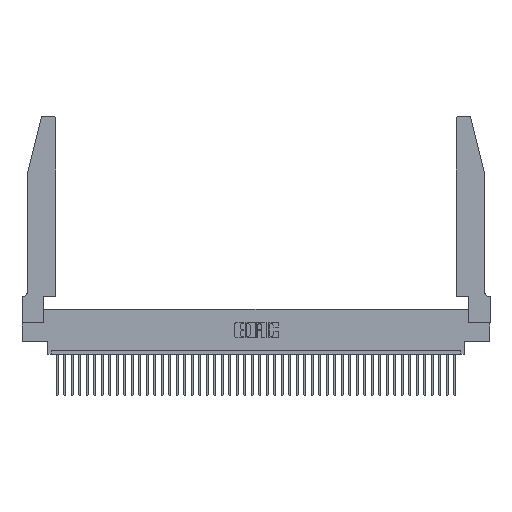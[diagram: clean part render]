
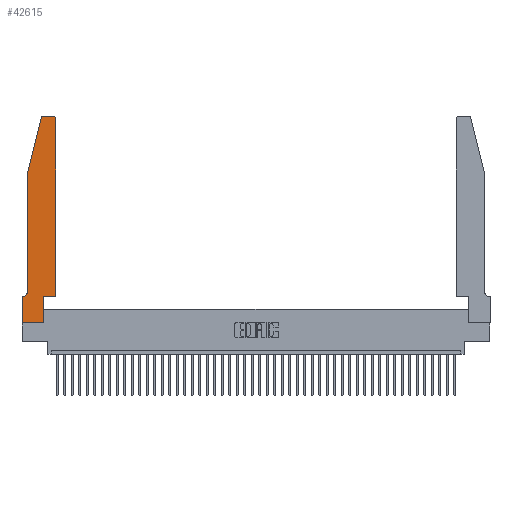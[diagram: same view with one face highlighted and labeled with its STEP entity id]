
A CAD part, top view. The second image highlights one B-rep face of the part: STEP entity #42615.
In plain terms, the highlighted planar face has unit normal (0, 0, 1).
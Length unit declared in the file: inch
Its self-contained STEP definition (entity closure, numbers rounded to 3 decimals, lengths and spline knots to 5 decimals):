
#697 = CARTESIAN_POINT ( 'NONE',  ( 0.0755, 2., 0.37 ) ) ;
#717 = VECTOR ( 'NONE', #19329, 39.37008 ) ;
#1772 = VECTOR ( 'NONE', #2911, 39.37008 ) ;
#1930 = VERTEX_POINT ( 'NONE', #11612 ) ;
#2911 = DIRECTION ( 'NONE',  ( 0., -1., 0. ) ) ;
#3520 = AXIS2_PLACEMENT_3D ( 'NONE', #26844, #40821, #43449 ) ;
#3695 = VERTEX_POINT ( 'NONE', #8639 ) ;
#3860 = EDGE_CURVE ( 'NONE', #17588, #12677, #14939, .T. ) ;
#5126 = CARTESIAN_POINT ( 'NONE',  ( 0., 0., 0.37 ) ) ;
#5827 = EDGE_LOOP ( 'NONE', ( #27876, #9896, #30669, #34247, #7781, #6226, #40055, #27131, #17702, #28849, #39138, #20513 ) ) ;
#5882 = DIRECTION ( 'NONE',  ( 0., 1., 0. ) ) ;
#6148 = CARTESIAN_POINT ( 'NONE',  ( 0., 0., 0.37 ) ) ;
#6226 = ORIENTED_EDGE ( 'NONE', *, *, #20479, .T. ) ;
#6521 = CARTESIAN_POINT ( 'NONE',  ( 0.25487, 2.72718, 0.37 ) ) ;
#7174 = CARTESIAN_POINT ( 'NONE',  ( 0.0755, 2., 0.37 ) ) ;
#7204 = DIRECTION ( 'NONE',  ( 1., 0., 0. ) ) ;
#7672 = EDGE_CURVE ( 'NONE', #11329, #1930, #38548, .T. ) ;
#7781 = ORIENTED_EDGE ( 'NONE', *, *, #15201, .T. ) ;
#8639 = CARTESIAN_POINT ( 'NONE',  ( 0.0055, 0.35, 0.37 ) ) ;
#8885 = CARTESIAN_POINT ( 'NONE',  ( 0.2865, 0.35, 0.37 ) ) ;
#9139 = EDGE_CURVE ( 'NONE', #18949, #39101, #30031, .T. ) ;
#9158 = EDGE_CURVE ( 'NONE', #14496, #18949, #19874, .T. ) ;
#9200 = CARTESIAN_POINT ( 'NONE',  ( 0.4505, 0.35, 0.37 ) ) ;
#9896 = ORIENTED_EDGE ( 'NONE', *, *, #11062, .T. ) ;
#10125 = EDGE_CURVE ( 'NONE', #12677, #40994, #11432, .T. ) ;
#10352 = DIRECTION ( 'NONE',  ( 1., 0., 0. ) ) ;
#11062 = EDGE_CURVE ( 'NONE', #21156, #11329, #23035, .T. ) ;
#11329 = VERTEX_POINT ( 'NONE', #6521 ) ;
#11432 = LINE ( 'NONE', #17126, #34320 ) ;
#11612 = CARTESIAN_POINT ( 'NONE',  ( 0.0755, 2., 0.37 ) ) ;
#12086 = DIRECTION ( 'NONE',  ( 0., 0., 1. ) ) ;
#12306 = LINE ( 'NONE', #38046, #34621 ) ;
#12342 = AXIS2_PLACEMENT_3D ( 'NONE', #22191, #12086, #29982 ) ;
#12677 = VERTEX_POINT ( 'NONE', #5126 ) ;
#13177 = CARTESIAN_POINT ( 'NONE',  ( 0.4205, 2.75, 0.37 ) ) ;
#14496 = VERTEX_POINT ( 'NONE', #18374 ) ;
#14939 = LINE ( 'NONE', #6148, #1772 ) ;
#15201 = EDGE_CURVE ( 'NONE', #42965, #3695, #32300, .T. ) ;
#16447 = DIRECTION ( 'NONE',  ( 1., 0., 0. ) ) ;
#16459 = EDGE_CURVE ( 'NONE', #20264, #14496, #19159, .T. ) ;
#16990 = DIRECTION ( 'NONE',  ( 0., 0., 1. ) ) ;
#17120 = PLANE ( 'NONE',  #40220 ) ;
#17126 = CARTESIAN_POINT ( 'NONE',  ( 0., 0., 0.37 ) ) ;
#17588 = VERTEX_POINT ( 'NONE', #36918 ) ;
#17645 = DIRECTION ( 'NONE',  ( -1., 0., 0. ) ) ;
#17702 = ORIENTED_EDGE ( 'NONE', *, *, #20177, .T. ) ;
#18374 = CARTESIAN_POINT ( 'NONE',  ( 0.4505, 0.35, 0.37 ) ) ;
#18949 = VERTEX_POINT ( 'NONE', #42520 ) ;
#19110 = CARTESIAN_POINT ( 'NONE',  ( 0.2865, 0., 0.37 ) ) ;
#19159 = LINE ( 'NONE', #9200, #21763 ) ;
#19329 = DIRECTION ( 'NONE',  ( 0., 1., 0. ) ) ;
#19874 = LINE ( 'NONE', #25463, #37877 ) ;
#20177 = EDGE_CURVE ( 'NONE', #40994, #20264, #26287, .T. ) ;
#20264 = VERTEX_POINT ( 'NONE', #8885 ) ;
#20285 = EDGE_CURVE ( 'NONE', #1930, #42965, #43249, .T. ) ;
#20479 = EDGE_CURVE ( 'NONE', #3695, #17588, #38376, .T. ) ;
#20513 = ORIENTED_EDGE ( 'NONE', *, *, #9139, .T. ) ;
#20932 = EDGE_CURVE ( 'NONE', #39101, #21156, #12306, .T. ) ;
#21156 = VERTEX_POINT ( 'NONE', #43833 ) ;
#21763 = VECTOR ( 'NONE', #7204, 39.37008 ) ;
#22191 = CARTESIAN_POINT ( 'NONE',  ( 0.4205, 2.72, 0.37 ) ) ;
#22979 = CARTESIAN_POINT ( 'NONE',  ( 0.0755, 0.42, 0.37 ) ) ;
#23007 = VECTOR ( 'NONE', #34397, 39.37008 ) ;
#23035 = CIRCLE ( 'NONE', #43161, 0.03 ) ;
#25463 = CARTESIAN_POINT ( 'NONE',  ( 0.4505, 0.35, 0.37 ) ) ;
#26287 = LINE ( 'NONE', #35855, #717 ) ;
#26844 = CARTESIAN_POINT ( 'NONE',  ( 0.0055, 0.42, 0.37 ) ) ;
#27131 = ORIENTED_EDGE ( 'NONE', *, *, #10125, .T. ) ;
#27876 = ORIENTED_EDGE ( 'NONE', *, *, #20932, .T. ) ;
#28679 = DIRECTION ( 'NONE',  ( -1., 0., 0. ) ) ;
#28849 = ORIENTED_EDGE ( 'NONE', *, *, #16459, .T. ) ;
#29982 = DIRECTION ( 'NONE',  ( 1., 0., 0. ) ) ;
#30031 = CIRCLE ( 'NONE', #12342, 0.03 ) ;
#30669 = ORIENTED_EDGE ( 'NONE', *, *, #7672, .T. ) ;
#30894 = CARTESIAN_POINT ( 'NONE',  ( 0., 0.35, 0.37 ) ) ;
#32300 = CIRCLE ( 'NONE', #3520, 0.07 ) ;
#33386 = DIRECTION ( 'NONE',  ( -0.239, -0.971, 0. ) ) ;
#34247 = ORIENTED_EDGE ( 'NONE', *, *, #20285, .T. ) ;
#34320 = VECTOR ( 'NONE', #10352, 39.37008 ) ;
#34397 = DIRECTION ( 'NONE',  ( 0., -1., 0. ) ) ;
#34621 = VECTOR ( 'NONE', #17645, 39.37008 ) ;
#34853 = VECTOR ( 'NONE', #33386, 39.37008 ) ;
#35855 = CARTESIAN_POINT ( 'NONE',  ( 0.2865, 0.35, 0.37 ) ) ;
#36858 = VECTOR ( 'NONE', #28679, 39.37008 ) ;
#36918 = CARTESIAN_POINT ( 'NONE',  ( 0., 0.35, 0.37 ) ) ;
#37681 = DIRECTION ( 'NONE',  ( 1., 0., 0. ) ) ;
#37877 = VECTOR ( 'NONE', #5882, 39.37008 ) ;
#38046 = CARTESIAN_POINT ( 'NONE',  ( 0.2605, 2.75, 0.37 ) ) ;
#38376 = LINE ( 'NONE', #42173, #36858 ) ;
#38548 = LINE ( 'NONE', #7174, #34853 ) ;
#39101 = VERTEX_POINT ( 'NONE', #13177 ) ;
#39138 = ORIENTED_EDGE ( 'NONE', *, *, #9158, .T. ) ;
#40055 = ORIENTED_EDGE ( 'NONE', *, *, #3860, .T. ) ;
#40220 = AXIS2_PLACEMENT_3D ( 'NONE', #30894, #16990, #37681 ) ;
#40293 = CARTESIAN_POINT ( 'NONE',  ( 0.284, 2.72, 0.37 ) ) ;
#40498 = FACE_OUTER_BOUND ( 'NONE', #5827, .T. ) ;
#40821 = DIRECTION ( 'NONE',  ( 0., 0., -1. ) ) ;
#40994 = VERTEX_POINT ( 'NONE', #19110 ) ;
#42173 = CARTESIAN_POINT ( 'NONE',  ( 0.0755, 0.35, 0.37 ) ) ;
#42520 = CARTESIAN_POINT ( 'NONE',  ( 0.4505, 2.72, 0.37 ) ) ;
#42615 = ADVANCED_FACE ( 'NONE', ( #40498 ), #17120, .T. ) ;
#42965 = VERTEX_POINT ( 'NONE', #22979 ) ;
#43161 = AXIS2_PLACEMENT_3D ( 'NONE', #40293, #43580, #16447 ) ;
#43249 = LINE ( 'NONE', #697, #23007 ) ;
#43449 = DIRECTION ( 'NONE',  ( -1., 0., 0. ) ) ;
#43580 = DIRECTION ( 'NONE',  ( 0., 0., 1. ) ) ;
#43833 = CARTESIAN_POINT ( 'NONE',  ( 0.284, 2.75, 0.37 ) ) ;
